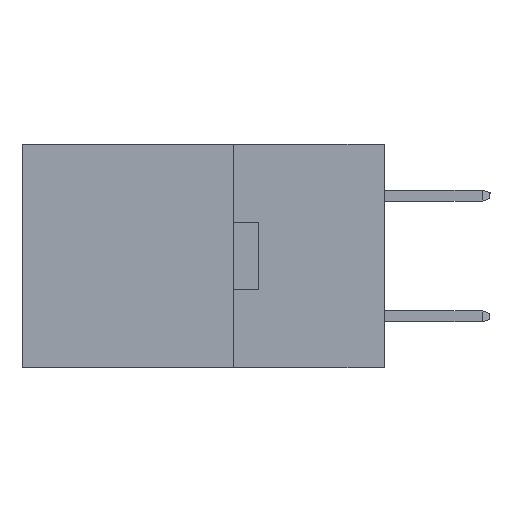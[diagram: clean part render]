
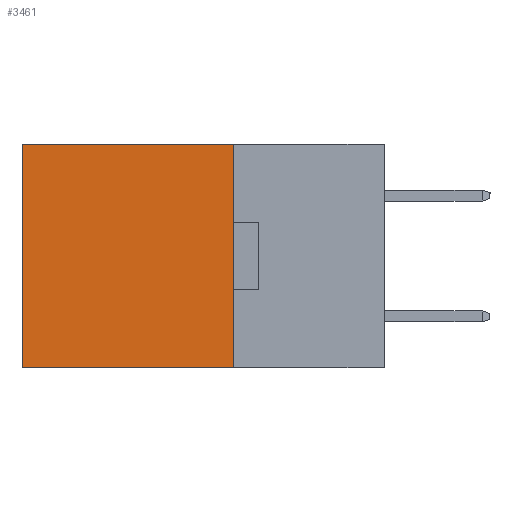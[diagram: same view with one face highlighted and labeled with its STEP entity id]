
A CAD part, left-side view. The second image highlights one B-rep face of the part: STEP entity #3461.
In plain terms, the highlighted planar face has unit normal (-1, 0, 0).
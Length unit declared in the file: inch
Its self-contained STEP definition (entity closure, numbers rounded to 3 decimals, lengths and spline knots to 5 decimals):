
#700 = CARTESIAN_POINT ( 'NONE',  ( 0.2615, 0.25, 0. ) ) ;
#772 = ORIENTED_EDGE ( 'NONE', *, *, #26623, .F. ) ;
#1782 = VECTOR ( 'NONE', #25002, 39.37008 ) ;
#1933 = LINE ( 'NONE', #2352, #13737 ) ;
#2352 = CARTESIAN_POINT ( 'NONE',  ( 0.2615, 0.25, -0.37 ) ) ;
#3461 = ADVANCED_FACE ( 'NONE', ( #15373 ), #10611, .F. ) ;
#4015 = CARTESIAN_POINT ( 'NONE',  ( 0.2615, 0.6, -0.37 ) ) ;
#4352 = EDGE_CURVE ( 'NONE', #7330, #26528, #1933, .T. ) ;
#4422 = CARTESIAN_POINT ( 'NONE',  ( 0.2615, 0.25, -0.37 ) ) ;
#5904 = CARTESIAN_POINT ( 'NONE',  ( 0.2615, 0.25, 0. ) ) ;
#6163 = CARTESIAN_POINT ( 'NONE',  ( 0.2615, 0.25, -0.37 ) ) ;
#7330 = VERTEX_POINT ( 'NONE', #4422 ) ;
#8037 = VECTOR ( 'NONE', #12800, 39.37008 ) ;
#8477 = DIRECTION ( 'NONE',  ( 0., 1., 0. ) ) ;
#8482 = VECTOR ( 'NONE', #17973, 39.37008 ) ;
#10326 = DIRECTION ( 'NONE',  ( 0., 0., -1. ) ) ;
#10611 = PLANE ( 'NONE',  #12243 ) ;
#11241 = ORIENTED_EDGE ( 'NONE', *, *, #4352, .F. ) ;
#11771 = VERTEX_POINT ( 'NONE', #700 ) ;
#12038 = LINE ( 'NONE', #22681, #8482 ) ;
#12210 = LINE ( 'NONE', #20421, #1782 ) ;
#12243 = AXIS2_PLACEMENT_3D ( 'NONE', #6163, #28134, #10326 ) ;
#12800 = DIRECTION ( 'NONE',  ( 0., 1., 0. ) ) ;
#13104 = ORIENTED_EDGE ( 'NONE', *, *, #23841, .T. ) ;
#13737 = VECTOR ( 'NONE', #8477, 39.37008 ) ;
#15373 = FACE_OUTER_BOUND ( 'NONE', #25384, .T. ) ;
#16739 = CARTESIAN_POINT ( 'NONE',  ( 0.2615, 0.6, 0. ) ) ;
#16843 = LINE ( 'NONE', #5904, #8037 ) ;
#17973 = DIRECTION ( 'NONE',  ( 0., 0., -1. ) ) ;
#20421 = CARTESIAN_POINT ( 'NONE',  ( 0.2615, 0.6, -0.37 ) ) ;
#20967 = EDGE_CURVE ( 'NONE', #11771, #25782, #16843, .T. ) ;
#22681 = CARTESIAN_POINT ( 'NONE',  ( 0.2615, 0.25, -0.37 ) ) ;
#23841 = EDGE_CURVE ( 'NONE', #25782, #26528, #12210, .T. ) ;
#25002 = DIRECTION ( 'NONE',  ( 0., 0., -1. ) ) ;
#25384 = EDGE_LOOP ( 'NONE', ( #13104, #11241, #772, #28272 ) ) ;
#25782 = VERTEX_POINT ( 'NONE', #16739 ) ;
#26528 = VERTEX_POINT ( 'NONE', #4015 ) ;
#26623 = EDGE_CURVE ( 'NONE', #11771, #7330, #12038, .T. ) ;
#28134 = DIRECTION ( 'NONE',  ( 1., 0., 0. ) ) ;
#28272 = ORIENTED_EDGE ( 'NONE', *, *, #20967, .T. ) ;
